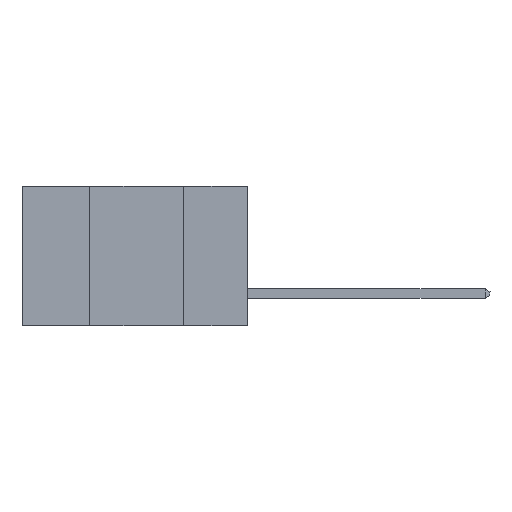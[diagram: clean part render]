
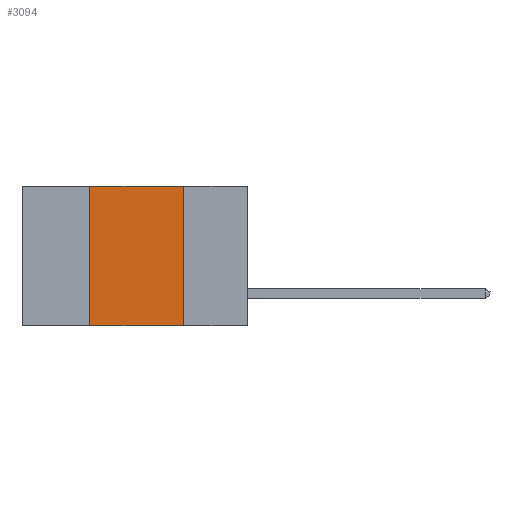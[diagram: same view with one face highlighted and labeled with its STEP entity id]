
A CAD part, left-side view. The second image highlights one B-rep face of the part: STEP entity #3094.
In plain terms, the highlighted planar face has unit normal (-1, 0, 0).
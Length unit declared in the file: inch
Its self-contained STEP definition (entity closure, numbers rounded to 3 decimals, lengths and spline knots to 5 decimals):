
#692 = PLANE ( 'NONE',  #4969 ) ;
#900 = VERTEX_POINT ( 'NONE', #4820 ) ;
#952 = CARTESIAN_POINT ( 'NONE',  ( 0., 0.17, -0.37 ) ) ;
#1593 = DIRECTION ( 'NONE',  ( 0., 0., -1. ) ) ;
#1980 = FACE_OUTER_BOUND ( 'NONE', #6863, .T. ) ;
#2292 = ORIENTED_EDGE ( 'NONE', *, *, #2537, .F. ) ;
#2456 = ORIENTED_EDGE ( 'NONE', *, *, #7700, .F. ) ;
#2503 = CARTESIAN_POINT ( 'NONE',  ( 0., 0.42, -0.37 ) ) ;
#2537 = EDGE_CURVE ( 'NONE', #4979, #900, #3951, .T. ) ;
#3094 = ADVANCED_FACE ( 'NONE', ( #1980 ), #692, .F. ) ;
#3419 = DIRECTION ( 'NONE',  ( 1., 0., 0. ) ) ;
#3538 = VERTEX_POINT ( 'NONE', #7333 ) ;
#3722 = LINE ( 'NONE', #4870, #4199 ) ;
#3790 = VECTOR ( 'NONE', #3831, 39.37008 ) ;
#3808 = EDGE_CURVE ( 'NONE', #3538, #7689, #6509, .T. ) ;
#3831 = DIRECTION ( 'NONE',  ( 0., -1., 0. ) ) ;
#3864 = CARTESIAN_POINT ( 'NONE',  ( 0., 0.6, 0. ) ) ;
#3866 = CARTESIAN_POINT ( 'NONE',  ( 0., 0.6, -0.37 ) ) ;
#3951 = LINE ( 'NONE', #3864, #3956 ) ;
#3956 = VECTOR ( 'NONE', #7069, 39.37008 ) ;
#4199 = VECTOR ( 'NONE', #1593, 39.37008 ) ;
#4616 = DIRECTION ( 'NONE',  ( 0., 0., 1. ) ) ;
#4820 = CARTESIAN_POINT ( 'NONE',  ( 0., 0.17, 0. ) ) ;
#4870 = CARTESIAN_POINT ( 'NONE',  ( 0., 0.17, -0.37 ) ) ;
#4969 = AXIS2_PLACEMENT_3D ( 'NONE', #7356, #3419, #5893 ) ;
#4979 = VERTEX_POINT ( 'NONE', #6102 ) ;
#5317 = ORIENTED_EDGE ( 'NONE', *, *, #5502, .F. ) ;
#5502 = EDGE_CURVE ( 'NONE', #3538, #4979, #5861, .T. ) ;
#5861 = LINE ( 'NONE', #2503, #6497 ) ;
#5893 = DIRECTION ( 'NONE',  ( 0., 0., -1. ) ) ;
#6102 = CARTESIAN_POINT ( 'NONE',  ( 0., 0.42, 0. ) ) ;
#6497 = VECTOR ( 'NONE', #4616, 39.37008 ) ;
#6509 = LINE ( 'NONE', #3866, #3790 ) ;
#6863 = EDGE_LOOP ( 'NONE', ( #2456, #2292, #5317, #7626 ) ) ;
#7069 = DIRECTION ( 'NONE',  ( 0., -1., 0. ) ) ;
#7333 = CARTESIAN_POINT ( 'NONE',  ( 0., 0.42, -0.37 ) ) ;
#7356 = CARTESIAN_POINT ( 'NONE',  ( 0., 0.6, 0. ) ) ;
#7626 = ORIENTED_EDGE ( 'NONE', *, *, #3808, .T. ) ;
#7689 = VERTEX_POINT ( 'NONE', #952 ) ;
#7700 = EDGE_CURVE ( 'NONE', #900, #7689, #3722, .T. ) ;
